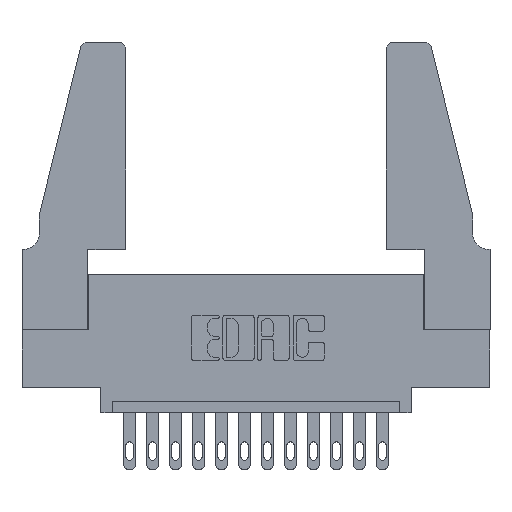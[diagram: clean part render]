
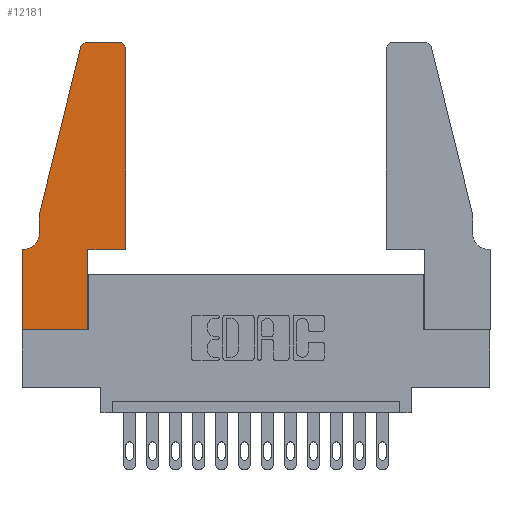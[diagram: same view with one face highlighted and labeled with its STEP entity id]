
A CAD part, top view. The second image highlights one B-rep face of the part: STEP entity #12181.
In plain terms, the highlighted planar face has unit normal (0, 0, 1).
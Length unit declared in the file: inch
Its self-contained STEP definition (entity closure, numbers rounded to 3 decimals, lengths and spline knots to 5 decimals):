
#211 = DIRECTION ( 'NONE',  ( 1., 0., 0. ) ) ;
#336 = CARTESIAN_POINT ( 'NONE',  ( 0., 0., 0.37 ) ) ;
#399 = DIRECTION ( 'NONE',  ( -1., 0., 0. ) ) ;
#400 = EDGE_CURVE ( 'NONE', #3760, #11240, #794, .T. ) ;
#456 = CARTESIAN_POINT ( 'NONE',  ( 0.0755, 0.35, 0.37 ) ) ;
#589 = VERTEX_POINT ( 'NONE', #13236 ) ;
#655 = EDGE_CURVE ( 'NONE', #15121, #9932, #8398, .T. ) ;
#776 = CARTESIAN_POINT ( 'NONE',  ( 0., 0.35, 0.37 ) ) ;
#794 = LINE ( 'NONE', #456, #2264 ) ;
#798 = DIRECTION ( 'NONE',  ( 0., 0., 1. ) ) ;
#964 = EDGE_CURVE ( 'NONE', #1786, #9104, #14260, .T. ) ;
#1124 = EDGE_CURVE ( 'NONE', #589, #3760, #12965, .T. ) ;
#1165 = EDGE_CURVE ( 'NONE', #2061, #1786, #5975, .T. ) ;
#1467 = CARTESIAN_POINT ( 'NONE',  ( 0.2865, 0.35, 0.37 ) ) ;
#1626 = AXIS2_PLACEMENT_3D ( 'NONE', #10244, #798, #12527 ) ;
#1786 = VERTEX_POINT ( 'NONE', #13631 ) ;
#1883 = CARTESIAN_POINT ( 'NONE',  ( 0.0755, 0.5, 0.37 ) ) ;
#2061 = VERTEX_POINT ( 'NONE', #5394 ) ;
#2264 = VECTOR ( 'NONE', #399, 39.37008 ) ;
#2664 = CARTESIAN_POINT ( 'NONE',  ( 0.0055, 0.42, 0.37 ) ) ;
#2947 = EDGE_CURVE ( 'NONE', #9932, #4674, #7598, .T. ) ;
#2982 = VECTOR ( 'NONE', #10597, 39.37008 ) ;
#3313 = DIRECTION ( 'NONE',  ( -1., 0., 0. ) ) ;
#3419 = CARTESIAN_POINT ( 'NONE',  ( 0.0055, 0.35, 0.37 ) ) ;
#3669 = ORIENTED_EDGE ( 'NONE', *, *, #10722, .T. ) ;
#3685 = VERTEX_POINT ( 'NONE', #12660 ) ;
#3760 = VERTEX_POINT ( 'NONE', #3419 ) ;
#3920 = DIRECTION ( 'NONE',  ( 1., 0., 0. ) ) ;
#4145 = DIRECTION ( 'NONE',  ( 1., 0., 0. ) ) ;
#4386 = ORIENTED_EDGE ( 'NONE', *, *, #655, .T. ) ;
#4502 = CARTESIAN_POINT ( 'NONE',  ( 0.2605, 1.25, 0.37 ) ) ;
#4585 = DIRECTION ( 'NONE',  ( 0., -1., 0. ) ) ;
#4674 = VERTEX_POINT ( 'NONE', #1883 ) ;
#4784 = CARTESIAN_POINT ( 'NONE',  ( 0.4505, 0.35, 0.37 ) ) ;
#5161 = DIRECTION ( 'NONE',  ( 0., 0., -1. ) ) ;
#5214 = DIRECTION ( 'NONE',  ( -1., 0., 0. ) ) ;
#5394 = CARTESIAN_POINT ( 'NONE',  ( 0.2865, 0.35, 0.37 ) ) ;
#5500 = ORIENTED_EDGE ( 'NONE', *, *, #11689, .T. ) ;
#5975 = LINE ( 'NONE', #13346, #8760 ) ;
#6151 = ORIENTED_EDGE ( 'NONE', *, *, #11309, .T. ) ;
#6158 = LINE ( 'NONE', #7816, #10959 ) ;
#6223 = EDGE_LOOP ( 'NONE', ( #10941, #4386, #9807, #8562, #6596, #15039, #11923, #3669, #5500, #7431, #10816, #6151 ) ) ;
#6500 = VECTOR ( 'NONE', #9266, 39.37008 ) ;
#6596 = ORIENTED_EDGE ( 'NONE', *, *, #1124, .T. ) ;
#7264 = CARTESIAN_POINT ( 'NONE',  ( 0.4505, 1.22, 0.37 ) ) ;
#7423 = DIRECTION ( 'NONE',  ( 0., 0., 1. ) ) ;
#7431 = ORIENTED_EDGE ( 'NONE', *, *, #1165, .T. ) ;
#7598 = LINE ( 'NONE', #13010, #6500 ) ;
#7792 = VECTOR ( 'NONE', #4585, 39.37008 ) ;
#7816 = CARTESIAN_POINT ( 'NONE',  ( 0., 0., 0.37 ) ) ;
#7985 = VECTOR ( 'NONE', #15072, 39.37008 ) ;
#8207 = DIRECTION ( 'NONE',  ( 1., 0., 0. ) ) ;
#8398 = CIRCLE ( 'NONE', #1626, 0.03 ) ;
#8411 = CARTESIAN_POINT ( 'NONE',  ( 0.4205, 1.22, 0.37 ) ) ;
#8562 = ORIENTED_EDGE ( 'NONE', *, *, #11951, .T. ) ;
#8704 = VERTEX_POINT ( 'NONE', #12433 ) ;
#8760 = VECTOR ( 'NONE', #3920, 39.37008 ) ;
#8807 = AXIS2_PLACEMENT_3D ( 'NONE', #8411, #10779, #211 ) ;
#8937 = CARTESIAN_POINT ( 'NONE',  ( 0.284, 1.25, 0.37 ) ) ;
#8953 = VECTOR ( 'NONE', #14387, 39.37008 ) ;
#9104 = VERTEX_POINT ( 'NONE', #7264 ) ;
#9223 = CARTESIAN_POINT ( 'NONE',  ( 0.0755, 0.5, 0.37 ) ) ;
#9266 = DIRECTION ( 'NONE',  ( -0.239, -0.971, 0. ) ) ;
#9446 = VECTOR ( 'NONE', #3313, 39.37008 ) ;
#9512 = PLANE ( 'NONE',  #11657 ) ;
#9807 = ORIENTED_EDGE ( 'NONE', *, *, #2947, .T. ) ;
#9932 = VERTEX_POINT ( 'NONE', #10501 ) ;
#10212 = LINE ( 'NONE', #9223, #7792 ) ;
#10230 = LINE ( 'NONE', #1467, #8953 ) ;
#10244 = CARTESIAN_POINT ( 'NONE',  ( 0.284, 1.22, 0.37 ) ) ;
#10369 = CARTESIAN_POINT ( 'NONE',  ( 0.2865, 0., 0.37 ) ) ;
#10501 = CARTESIAN_POINT ( 'NONE',  ( 0.25487, 1.22718, 0.37 ) ) ;
#10539 = CARTESIAN_POINT ( 'NONE',  ( 0., 0.35, 0.37 ) ) ;
#10597 = DIRECTION ( 'NONE',  ( 0., 1., 0. ) ) ;
#10722 = EDGE_CURVE ( 'NONE', #3685, #13084, #6158, .T. ) ;
#10779 = DIRECTION ( 'NONE',  ( 0., 0., 1. ) ) ;
#10816 = ORIENTED_EDGE ( 'NONE', *, *, #964, .T. ) ;
#10941 = ORIENTED_EDGE ( 'NONE', *, *, #13143, .T. ) ;
#10959 = VECTOR ( 'NONE', #4145, 39.37008 ) ;
#11240 = VERTEX_POINT ( 'NONE', #776 ) ;
#11309 = EDGE_CURVE ( 'NONE', #9104, #8704, #12943, .T. ) ;
#11657 = AXIS2_PLACEMENT_3D ( 'NONE', #10539, #7423, #8207 ) ;
#11689 = EDGE_CURVE ( 'NONE', #13084, #2061, #10230, .T. ) ;
#11749 = EDGE_CURVE ( 'NONE', #11240, #3685, #14793, .T. ) ;
#11923 = ORIENTED_EDGE ( 'NONE', *, *, #11749, .T. ) ;
#11949 = AXIS2_PLACEMENT_3D ( 'NONE', #2664, #5161, #5214 ) ;
#11951 = EDGE_CURVE ( 'NONE', #4674, #589, #10212, .T. ) ;
#12181 = ADVANCED_FACE ( 'NONE', ( #13875 ), #9512, .T. ) ;
#12433 = CARTESIAN_POINT ( 'NONE',  ( 0.4205, 1.25, 0.37 ) ) ;
#12527 = DIRECTION ( 'NONE',  ( 1., 0., 0. ) ) ;
#12545 = LINE ( 'NONE', #4502, #9446 ) ;
#12660 = CARTESIAN_POINT ( 'NONE',  ( 0., 0., 0.37 ) ) ;
#12943 = CIRCLE ( 'NONE', #8807, 0.03 ) ;
#12965 = CIRCLE ( 'NONE', #11949, 0.07 ) ;
#13010 = CARTESIAN_POINT ( 'NONE',  ( 0.0755, 0.5, 0.37 ) ) ;
#13084 = VERTEX_POINT ( 'NONE', #10369 ) ;
#13143 = EDGE_CURVE ( 'NONE', #8704, #15121, #12545, .T. ) ;
#13236 = CARTESIAN_POINT ( 'NONE',  ( 0.0755, 0.42, 0.37 ) ) ;
#13346 = CARTESIAN_POINT ( 'NONE',  ( 0.4505, 0.35, 0.37 ) ) ;
#13631 = CARTESIAN_POINT ( 'NONE',  ( 0.4505, 0.35, 0.37 ) ) ;
#13875 = FACE_OUTER_BOUND ( 'NONE', #6223, .T. ) ;
#14260 = LINE ( 'NONE', #4784, #2982 ) ;
#14387 = DIRECTION ( 'NONE',  ( 0., 1., 0. ) ) ;
#14793 = LINE ( 'NONE', #336, #7985 ) ;
#15039 = ORIENTED_EDGE ( 'NONE', *, *, #400, .T. ) ;
#15072 = DIRECTION ( 'NONE',  ( 0., -1., 0. ) ) ;
#15121 = VERTEX_POINT ( 'NONE', #8937 ) ;
